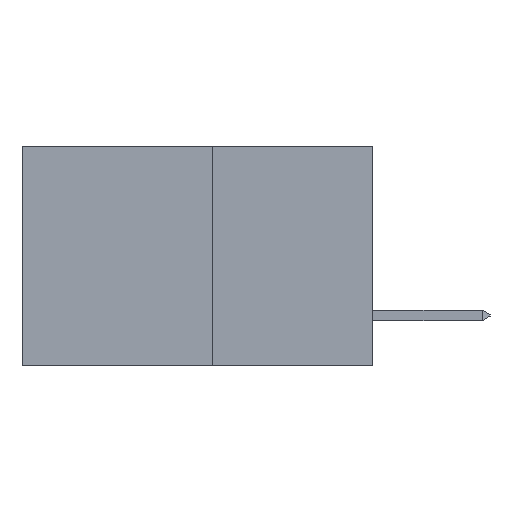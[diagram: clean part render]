
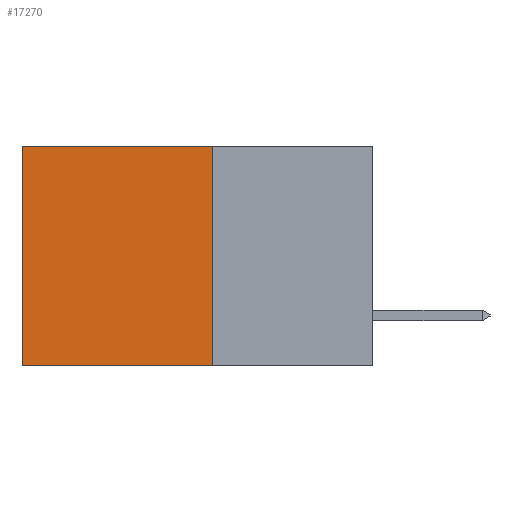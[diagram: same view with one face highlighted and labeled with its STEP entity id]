
A CAD part, left-side view. The second image highlights one B-rep face of the part: STEP entity #17270.
In plain terms, the highlighted planar face has unit normal (-1, 0, 0).
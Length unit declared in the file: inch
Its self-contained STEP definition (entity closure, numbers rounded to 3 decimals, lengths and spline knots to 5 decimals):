
#2 = LINE ( 'NONE', #9528, #3809 ) ;
#1228 = DIRECTION ( 'NONE',  ( 0., 0., -1. ) ) ;
#1772 = CARTESIAN_POINT ( 'NONE',  ( 0.277, 0.27, -0.37 ) ) ;
#1790 = VERTEX_POINT ( 'NONE', #17197 ) ;
#1832 = PLANE ( 'NONE',  #2537 ) ;
#2315 = EDGE_CURVE ( 'NONE', #4404, #17804, #2, .T. ) ;
#2537 = AXIS2_PLACEMENT_3D ( 'NONE', #1772, #3443, #14800 ) ;
#3224 = CARTESIAN_POINT ( 'NONE',  ( 0.277, 0.59, -0.37 ) ) ;
#3443 = DIRECTION ( 'NONE',  ( 1., 0., 0. ) ) ;
#3809 = VECTOR ( 'NONE', #1228, 39.37008 ) ;
#4027 = VECTOR ( 'NONE', #18336, 39.37008 ) ;
#4404 = VERTEX_POINT ( 'NONE', #17207 ) ;
#7032 = CARTESIAN_POINT ( 'NONE',  ( 0.277, 0.27, -0.37 ) ) ;
#7125 = CARTESIAN_POINT ( 'NONE',  ( 0.277, 0.27, 0. ) ) ;
#8311 = ORIENTED_EDGE ( 'NONE', *, *, #2315, .T. ) ;
#8565 = EDGE_CURVE ( 'NONE', #20533, #1790, #11477, .T. ) ;
#9528 = CARTESIAN_POINT ( 'NONE',  ( 0.277, 0.59, -0.37 ) ) ;
#11477 = LINE ( 'NONE', #15472, #19484 ) ;
#11833 = LINE ( 'NONE', #7125, #19839 ) ;
#11951 = EDGE_CURVE ( 'NONE', #20533, #4404, #11833, .T. ) ;
#12814 = ORIENTED_EDGE ( 'NONE', *, *, #16204, .F. ) ;
#13213 = ORIENTED_EDGE ( 'NONE', *, *, #11951, .T. ) ;
#13450 = CARTESIAN_POINT ( 'NONE',  ( 0.277, 0.27, 0. ) ) ;
#13703 = EDGE_LOOP ( 'NONE', ( #8311, #12814, #14992, #13213 ) ) ;
#14800 = DIRECTION ( 'NONE',  ( 0., 0., -1. ) ) ;
#14992 = ORIENTED_EDGE ( 'NONE', *, *, #8565, .F. ) ;
#15472 = CARTESIAN_POINT ( 'NONE',  ( 0.277, 0.27, -0.37 ) ) ;
#16204 = EDGE_CURVE ( 'NONE', #1790, #17804, #16459, .T. ) ;
#16459 = LINE ( 'NONE', #7032, #4027 ) ;
#16657 = FACE_OUTER_BOUND ( 'NONE', #13703, .T. ) ;
#16839 = DIRECTION ( 'NONE',  ( 0., 1., 0. ) ) ;
#17084 = DIRECTION ( 'NONE',  ( 0., 0., -1. ) ) ;
#17197 = CARTESIAN_POINT ( 'NONE',  ( 0.277, 0.27, -0.37 ) ) ;
#17207 = CARTESIAN_POINT ( 'NONE',  ( 0.277, 0.59, 0. ) ) ;
#17270 = ADVANCED_FACE ( 'NONE', ( #16657 ), #1832, .F. ) ;
#17804 = VERTEX_POINT ( 'NONE', #3224 ) ;
#18336 = DIRECTION ( 'NONE',  ( 0., 1., 0. ) ) ;
#19484 = VECTOR ( 'NONE', #17084, 39.37008 ) ;
#19839 = VECTOR ( 'NONE', #16839, 39.37008 ) ;
#20533 = VERTEX_POINT ( 'NONE', #13450 ) ;
